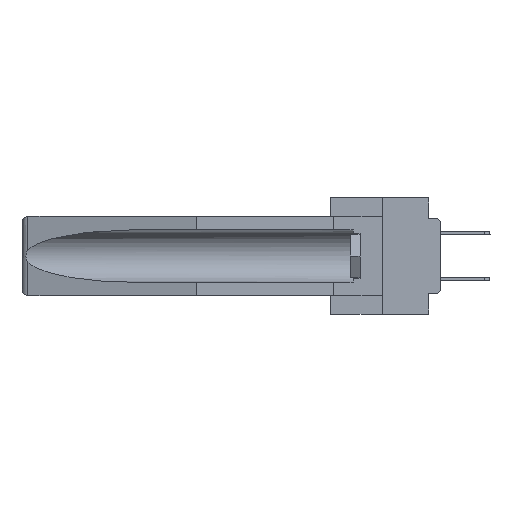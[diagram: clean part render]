
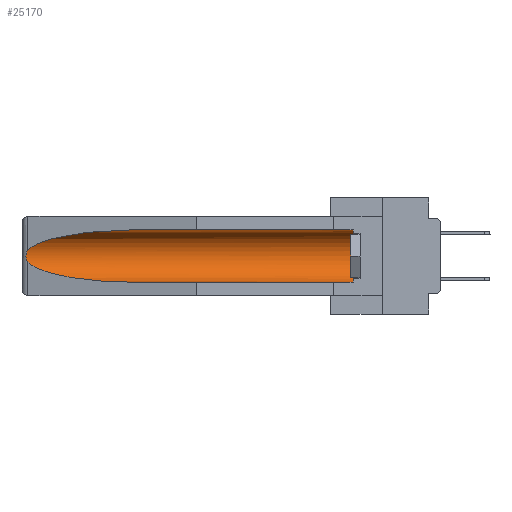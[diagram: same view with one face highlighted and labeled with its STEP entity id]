
A CAD part, left-side view. The second image highlights one B-rep face of the part: STEP entity #25170.
In plain terms, the highlighted cylindrical face has radius 2.857 mm (diameter 5.715 mm), a partial arc.
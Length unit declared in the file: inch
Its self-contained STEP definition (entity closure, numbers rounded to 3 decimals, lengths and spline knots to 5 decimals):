
#622 = CARTESIAN_POINT ( 'NONE',  ( 0.21114, 1.30732, -0.284 ) ) ;
#882 = AXIS2_PLACEMENT_3D ( 'NONE', #22209, #24791, #19278 ) ;
#1255 =( BOUNDED_CURVE ( )  B_SPLINE_CURVE ( 3, ( #13389, #3268, #622, #31433 ),
 .UNSPECIFIED., .F., .F. ) 
 B_SPLINE_CURVE_WITH_KNOTS ( ( 4, 4 ),
 ( 0.1948, 1.5708 ),
 .UNSPECIFIED. ) 
 CURVE ( )  GEOMETRIC_REPRESENTATION_ITEM ( )  RATIONAL_B_SPLINE_CURVE ( ( 1., 0.848, 0.848, 1. ) ) 
 REPRESENTATION_ITEM ( '' )  );
#1887 = CARTESIAN_POINT ( 'NONE',  ( 0.155, 1.07973, -0.059 ) ) ;
#2104 = CARTESIAN_POINT ( 'NONE',  ( 0.26537, 1.52718, -0.14972 ) ) ;
#2396 = CARTESIAN_POINT ( 'NONE',  ( 0.26537, 1.52718, -0.14972 ) ) ;
#2658 = EDGE_CURVE ( 'NONE', #21584, #15022, #1255, .T. ) ;
#3268 = CARTESIAN_POINT ( 'NONE',  ( 0.25451, 1.48313, -0.24835 ) ) ;
#3297 = VERTEX_POINT ( 'NONE', #7652 ) ;
#4313 = EDGE_CURVE ( 'NONE', #16238, #3297, #11665, .T. ) ;
#4704 = EDGE_CURVE ( 'NONE', #3297, #6887, #5942, .T. ) ;
#4880 = CARTESIAN_POINT ( 'NONE',  ( 0.26537, 1.52718, -0.19328 ) ) ;
#4919 = EDGE_LOOP ( 'NONE', ( #15904, #25268, #14986, #13453, #12447, #12458 ) ) ;
#5225 = CARTESIAN_POINT ( 'NONE',  ( 0.2675, 1.53308, -0.17534 ) ) ;
#5942 = LINE ( 'NONE', #29664, #16179 ) ;
#6887 = VERTEX_POINT ( 'NONE', #20949 ) ;
#7117 = DIRECTION ( 'NONE',  ( 0., 0., 1. ) ) ;
#7502 = CARTESIAN_POINT ( 'NONE',  ( 0.2675, 1.53308, -0.16763 ) ) ;
#7652 = CARTESIAN_POINT ( 'NONE',  ( 0.155, 0.126, -0.059 ) ) ;
#7741 = EDGE_CURVE ( 'NONE', #6887, #19328, #28947, .T. ) ;
#10056 = EDGE_CURVE ( 'NONE', #19328, #21584, #23760, .T. ) ;
#10110 = CARTESIAN_POINT ( 'NONE',  ( 0.26655, 1.53094, -0.18657 ) ) ;
#11665 = CIRCLE ( 'NONE', #16249, 0.1125 ) ;
#11691 = LINE ( 'NONE', #17401, #30351 ) ;
#11945 = DIRECTION ( 'NONE',  ( 0., 1., 0. ) ) ;
#12447 = ORIENTED_EDGE ( 'NONE', *, *, #4313, .T. ) ;
#12458 = ORIENTED_EDGE ( 'NONE', *, *, #4704, .T. ) ;
#12618 = CARTESIAN_POINT ( 'NONE',  ( 0.2673, 1.5327, -0.16383 ) ) ;
#12846 = CARTESIAN_POINT ( 'NONE',  ( 0.26597, 1.5296, -0.19026 ) ) ;
#13389 = CARTESIAN_POINT ( 'NONE',  ( 0.26537, 1.52718, -0.19328 ) ) ;
#13453 = ORIENTED_EDGE ( 'NONE', *, *, #17991, .F. ) ;
#14986 = ORIENTED_EDGE ( 'NONE', *, *, #2658, .T. ) ;
#15022 = VERTEX_POINT ( 'NONE', #15533 ) ;
#15351 = FACE_OUTER_BOUND ( 'NONE', #4919, .T. ) ;
#15489 = CARTESIAN_POINT ( 'NONE',  ( 0.26537, 1.52718, -0.14972 ) ) ;
#15533 = CARTESIAN_POINT ( 'NONE',  ( 0.155, 1.07973, -0.284 ) ) ;
#15904 = ORIENTED_EDGE ( 'NONE', *, *, #7741, .T. ) ;
#16179 = VECTOR ( 'NONE', #11945, 39.37008 ) ;
#16238 = VERTEX_POINT ( 'NONE', #25908 ) ;
#16249 = AXIS2_PLACEMENT_3D ( 'NONE', #22455, #22779, #7117 ) ;
#16353 = CARTESIAN_POINT ( 'NONE',  ( 0.26537, 1.52718, -0.19328 ) ) ;
#17401 = CARTESIAN_POINT ( 'NONE',  ( 0.155, -0.30754, -0.284 ) ) ;
#17991 = EDGE_CURVE ( 'NONE', #16238, #15022, #11691, .T. ) ;
#18324 = CARTESIAN_POINT ( 'NONE',  ( 0.2673, 1.53269, -0.17917 ) ) ;
#19278 = DIRECTION ( 'NONE',  ( 0., 0., 1. ) ) ;
#19328 = VERTEX_POINT ( 'NONE', #15489 ) ;
#20188 = CARTESIAN_POINT ( 'NONE',  ( 0.25451, 1.48313, -0.09465 ) ) ;
#20949 = CARTESIAN_POINT ( 'NONE',  ( 0.155, 1.07973, -0.059 ) ) ;
#21584 = VERTEX_POINT ( 'NONE', #16353 ) ;
#22209 = CARTESIAN_POINT ( 'NONE',  ( 0.155, -0.30754, -0.1715 ) ) ;
#22455 = CARTESIAN_POINT ( 'NONE',  ( 0.155, 0.126, -0.1715 ) ) ;
#22779 = DIRECTION ( 'NONE',  ( 0., -1., 0. ) ) ;
#23760 = B_SPLINE_CURVE_WITH_KNOTS ( 'NONE', 3,
 ( #2396, #33624, #33391, #12618, #7502, #5225, #18324, #10110, #12846, #4880 ),
 .UNSPECIFIED., .F., .F.,
 ( 4, 2, 2, 2, 4 ),
 ( 0., 0.00029, 0.00058, 0.00087, 0.00117 ),
 .UNSPECIFIED. ) ;
#24791 = DIRECTION ( 'NONE',  ( 0., 1., 0. ) ) ;
#25170 = ADVANCED_FACE ( 'NONE', ( #15351 ), #27530, .F. ) ;
#25268 = ORIENTED_EDGE ( 'NONE', *, *, #10056, .T. ) ;
#25908 = CARTESIAN_POINT ( 'NONE',  ( 0.155, 0.126, -0.284 ) ) ;
#27482 = DIRECTION ( 'NONE',  ( 0., 1., 0. ) ) ;
#27530 = CYLINDRICAL_SURFACE ( 'NONE', #882, 0.1125 ) ;
#28947 =( BOUNDED_CURVE ( )  B_SPLINE_CURVE ( 3, ( #1887, #33116, #20188, #2104 ),
 .UNSPECIFIED., .F., .F. ) 
 B_SPLINE_CURVE_WITH_KNOTS ( ( 4, 4 ),
 ( 4.71239, 6.08839 ),
 .UNSPECIFIED. ) 
 CURVE ( )  GEOMETRIC_REPRESENTATION_ITEM ( )  RATIONAL_B_SPLINE_CURVE ( ( 1., 0.848, 0.848, 1. ) ) 
 REPRESENTATION_ITEM ( '' )  );
#29664 = CARTESIAN_POINT ( 'NONE',  ( 0.155, -0.30754, -0.059 ) ) ;
#30351 = VECTOR ( 'NONE', #27482, 39.37008 ) ;
#31433 = CARTESIAN_POINT ( 'NONE',  ( 0.155, 1.07973, -0.284 ) ) ;
#33116 = CARTESIAN_POINT ( 'NONE',  ( 0.21114, 1.30732, -0.059 ) ) ;
#33391 = CARTESIAN_POINT ( 'NONE',  ( 0.26654, 1.53092, -0.15636 ) ) ;
#33624 = CARTESIAN_POINT ( 'NONE',  ( 0.26597, 1.52961, -0.15275 ) ) ;
